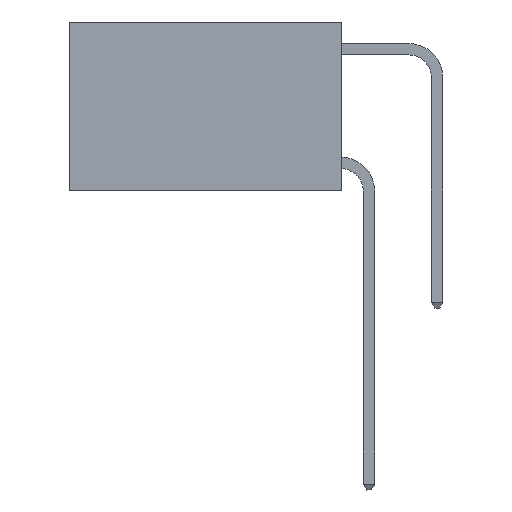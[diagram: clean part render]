
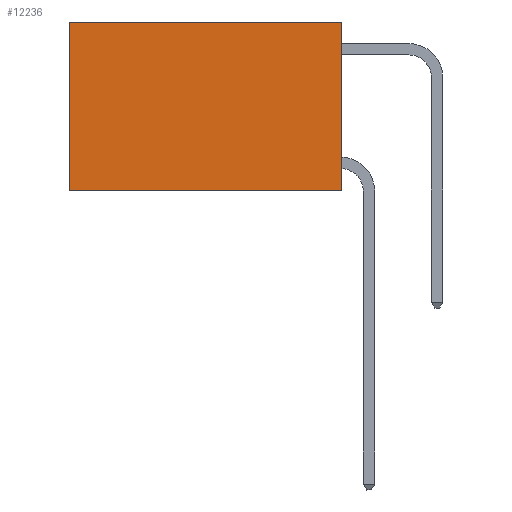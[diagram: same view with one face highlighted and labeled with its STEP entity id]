
A CAD part, left-side view. The second image highlights one B-rep face of the part: STEP entity #12236.
In plain terms, the highlighted planar face has unit normal (-1, 0, 0).
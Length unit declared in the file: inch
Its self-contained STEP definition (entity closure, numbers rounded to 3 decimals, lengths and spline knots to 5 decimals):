
#34 = ORIENTED_EDGE ( 'NONE', *, *, #11119, .T. ) ;
#506 = LINE ( 'NONE', #9917, #11966 ) ;
#865 = LINE ( 'NONE', #10848, #1221 ) ;
#911 = CARTESIAN_POINT ( 'NONE',  ( 0.2625, 0., -0.37 ) ) ;
#962 = CARTESIAN_POINT ( 'NONE',  ( 0.2625, 0.6, 0. ) ) ;
#1221 = VECTOR ( 'NONE', #3165, 39.37008 ) ;
#2074 = AXIS2_PLACEMENT_3D ( 'NONE', #11424, #12557, #5974 ) ;
#2750 = EDGE_LOOP ( 'NONE', ( #14151, #6341, #5600, #34 ) ) ;
#3165 = DIRECTION ( 'NONE',  ( 0., 0., -1. ) ) ;
#3494 = DIRECTION ( 'NONE',  ( 0., 1., 0. ) ) ;
#3550 = EDGE_CURVE ( 'NONE', #5984, #6934, #13743, .T. ) ;
#4530 = DIRECTION ( 'NONE',  ( 0., 1., 0. ) ) ;
#4632 = CARTESIAN_POINT ( 'NONE',  ( 0.2625, 0., -0.37 ) ) ;
#5054 = EDGE_CURVE ( 'NONE', #10988, #6934, #5751, .T. ) ;
#5600 = ORIENTED_EDGE ( 'NONE', *, *, #11527, .F. ) ;
#5751 = LINE ( 'NONE', #4632, #11229 ) ;
#5974 = DIRECTION ( 'NONE',  ( 0., 0., -1. ) ) ;
#5984 = VERTEX_POINT ( 'NONE', #7573 ) ;
#6341 = ORIENTED_EDGE ( 'NONE', *, *, #5054, .F. ) ;
#6934 = VERTEX_POINT ( 'NONE', #12609 ) ;
#7573 = CARTESIAN_POINT ( 'NONE',  ( 0.2625, 0.6, 0. ) ) ;
#8846 = VERTEX_POINT ( 'NONE', #10598 ) ;
#9233 = PLANE ( 'NONE',  #2074 ) ;
#9917 = CARTESIAN_POINT ( 'NONE',  ( 0.2625, 0., 0. ) ) ;
#10598 = CARTESIAN_POINT ( 'NONE',  ( 0.2625, 0., 0. ) ) ;
#10848 = CARTESIAN_POINT ( 'NONE',  ( 0.2625, 0., 0. ) ) ;
#10988 = VERTEX_POINT ( 'NONE', #911 ) ;
#11119 = EDGE_CURVE ( 'NONE', #8846, #5984, #506, .T. ) ;
#11229 = VECTOR ( 'NONE', #3494, 39.37008 ) ;
#11424 = CARTESIAN_POINT ( 'NONE',  ( 0.2625, 0., 0. ) ) ;
#11527 = EDGE_CURVE ( 'NONE', #8846, #10988, #865, .T. ) ;
#11966 = VECTOR ( 'NONE', #4530, 39.37008 ) ;
#12236 = ADVANCED_FACE ( 'NONE', ( #13302 ), #9233, .F. ) ;
#12557 = DIRECTION ( 'NONE',  ( 1., 0., 0. ) ) ;
#12609 = CARTESIAN_POINT ( 'NONE',  ( 0.2625, 0.6, -0.37 ) ) ;
#13302 = FACE_OUTER_BOUND ( 'NONE', #2750, .T. ) ;
#13394 = VECTOR ( 'NONE', #14272, 39.37008 ) ;
#13743 = LINE ( 'NONE', #962, #13394 ) ;
#14151 = ORIENTED_EDGE ( 'NONE', *, *, #3550, .T. ) ;
#14272 = DIRECTION ( 'NONE',  ( 0., 0., -1. ) ) ;
